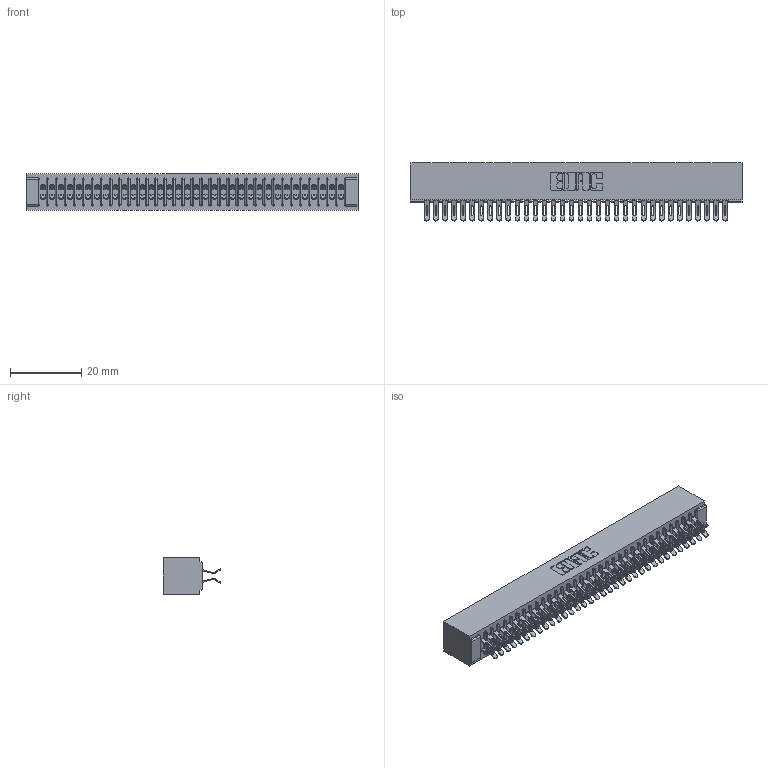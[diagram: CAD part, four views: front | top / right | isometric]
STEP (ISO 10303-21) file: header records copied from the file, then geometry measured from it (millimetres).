
FILE_DESCRIPTION (( 'STEP AP203' ), '1' );
FILE_NAME ('391-068-555-201.STEP', '2018-08-09T13:49:41', ( '' ), ( '' ), 'SwSTEP 2.0', 'SolidWorks 2016', '' );
FILE_SCHEMA (( 'CONFIG_CONTROL_DESIGN' ));
Length unit declared in the file: inch
Products named in the file (3): 391-068-555-201; 341 Part_No Mounting Lugs; 341-292-001_341-292-155
Assembly tree (69 placements, depth 2):
  391-068-555-201
    341 Part_No Mounting Lugs
    341-292-001_341-292-155  x68
Bounding box: 93.34 x 16.31 x 10.16 mm (x, y, z)
Volume: 7208.3 mm3; surface area: 13760.2 mm2
Topology: 69 solids, 69 shells, 5412 faces, 16170 edges, 10526 vertices
Faces by surface type: plane 2920, cylinder 2356, sphere 70, torus 66
Entity records: 42405 total; most frequent: CARTESIAN_POINT 7064, ORIENTED_EDGE 7008, DIRECTION 6850, EDGE_CURVE 3504, VECTOR 2810, LINE 2810, VERTEX_POINT 2218, AXIS2_PLACEMENT_3D 2020
